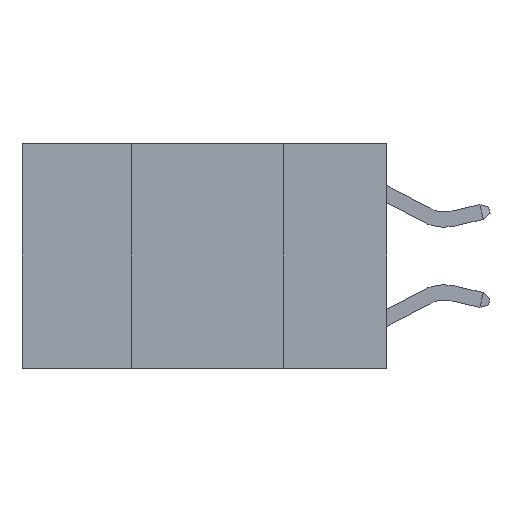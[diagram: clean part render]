
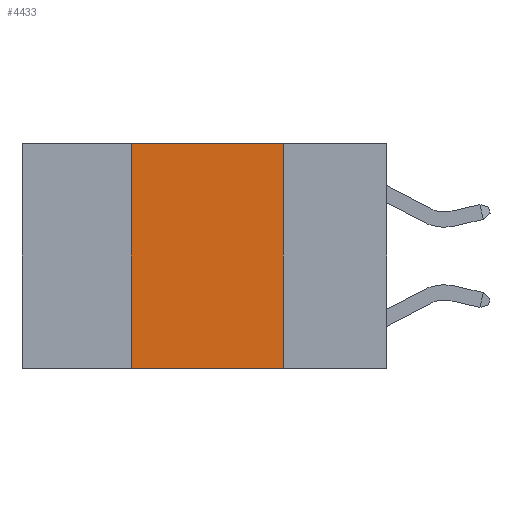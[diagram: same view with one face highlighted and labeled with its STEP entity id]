
A CAD part, left-side view. The second image highlights one B-rep face of the part: STEP entity #4433.
In plain terms, the highlighted planar face has unit normal (-1, 0, 0).
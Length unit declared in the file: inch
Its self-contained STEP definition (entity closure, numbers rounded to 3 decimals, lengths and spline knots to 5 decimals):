
#121 = VERTEX_POINT ( 'NONE', #5608 ) ;
#158 = CARTESIAN_POINT ( 'NONE',  ( 0., 0.42, -0.37 ) ) ;
#960 = DIRECTION ( 'NONE',  ( 0., -1., 0. ) ) ;
#1042 = LINE ( 'NONE', #6382, #6301 ) ;
#1396 = VECTOR ( 'NONE', #6828, 39.37008 ) ;
#1512 = FACE_OUTER_BOUND ( 'NONE', #8513, .T. ) ;
#1944 = LINE ( 'NONE', #4046, #1396 ) ;
#2805 = DIRECTION ( 'NONE',  ( 1., 0., 0. ) ) ;
#3047 = DIRECTION ( 'NONE',  ( 0., -1., 0. ) ) ;
#3286 = VERTEX_POINT ( 'NONE', #7819 ) ;
#3415 = PLANE ( 'NONE',  #4748 ) ;
#4046 = CARTESIAN_POINT ( 'NONE',  ( 0., 0.42, 0. ) ) ;
#4056 = CARTESIAN_POINT ( 'NONE',  ( 0., 0.6, -0.37 ) ) ;
#4102 = EDGE_CURVE ( 'NONE', #6137, #3286, #1042, .T. ) ;
#4207 = VECTOR ( 'NONE', #960, 39.37008 ) ;
#4433 = ADVANCED_FACE ( 'NONE', ( #1512 ), #3415, .F. ) ;
#4748 = AXIS2_PLACEMENT_3D ( 'NONE', #7427, #2805, #5475 ) ;
#4780 = ORIENTED_EDGE ( 'NONE', *, *, #4102, .F. ) ;
#4915 = ORIENTED_EDGE ( 'NONE', *, *, #5564, .F. ) ;
#5182 = VECTOR ( 'NONE', #7188, 39.37008 ) ;
#5277 = LINE ( 'NONE', #6460, #5182 ) ;
#5378 = EDGE_CURVE ( 'NONE', #7789, #121, #6229, .T. ) ;
#5475 = DIRECTION ( 'NONE',  ( 0., 0., -1. ) ) ;
#5564 = EDGE_CURVE ( 'NONE', #7789, #6137, #1944, .T. ) ;
#5608 = CARTESIAN_POINT ( 'NONE',  ( 0., 0.17, -0.37 ) ) ;
#5783 = EDGE_CURVE ( 'NONE', #3286, #121, #5277, .T. ) ;
#6137 = VERTEX_POINT ( 'NONE', #7499 ) ;
#6229 = LINE ( 'NONE', #4056, #4207 ) ;
#6301 = VECTOR ( 'NONE', #3047, 39.37008 ) ;
#6382 = CARTESIAN_POINT ( 'NONE',  ( 0., 0.6, 0. ) ) ;
#6460 = CARTESIAN_POINT ( 'NONE',  ( 0., 0.17, 0. ) ) ;
#6828 = DIRECTION ( 'NONE',  ( 0., 0., 1. ) ) ;
#7188 = DIRECTION ( 'NONE',  ( 0., 0., -1. ) ) ;
#7427 = CARTESIAN_POINT ( 'NONE',  ( 0., 0.6, 0. ) ) ;
#7499 = CARTESIAN_POINT ( 'NONE',  ( 0., 0.42, 0. ) ) ;
#7558 = ORIENTED_EDGE ( 'NONE', *, *, #5783, .F. ) ;
#7789 = VERTEX_POINT ( 'NONE', #158 ) ;
#7819 = CARTESIAN_POINT ( 'NONE',  ( 0., 0.17, 0. ) ) ;
#8513 = EDGE_LOOP ( 'NONE', ( #7558, #4780, #4915, #8621 ) ) ;
#8621 = ORIENTED_EDGE ( 'NONE', *, *, #5378, .T. ) ;
